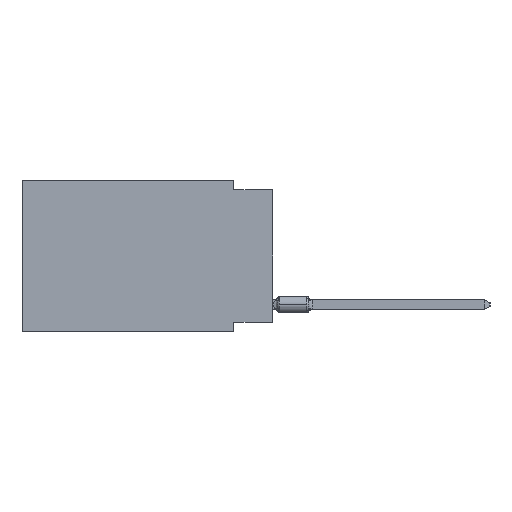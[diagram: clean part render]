
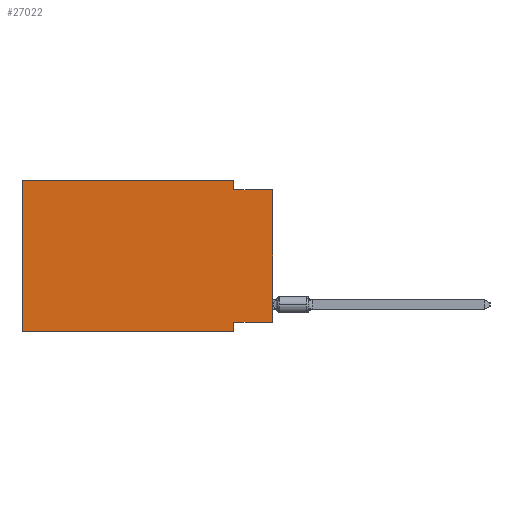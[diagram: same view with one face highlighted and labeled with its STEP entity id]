
A CAD part, left-side view. The second image highlights one B-rep face of the part: STEP entity #27022.
In plain terms, the highlighted planar face has unit normal (-1, 0, 0).
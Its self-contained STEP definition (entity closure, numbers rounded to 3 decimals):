
#645 = VERTEX_POINT ( 'NONE', #24655 ) ;
#1365 = CARTESIAN_POINT ( 'NONE',  ( 0., 0., -0.635 ) ) ;
#2185 = CARTESIAN_POINT ( 'NONE',  ( 0., 0., -0.635 ) ) ;
#3046 = LINE ( 'NONE', #20510, #38829 ) ;
#3589 = VERTEX_POINT ( 'NONE', #34357 ) ;
#4240 = DIRECTION ( 'NONE',  ( 0., 0., -1. ) ) ;
#5057 = DIRECTION ( 'NONE',  ( 0., -1., 0. ) ) ;
#5814 = LINE ( 'NONE', #32016, #23942 ) ;
#8572 = ORIENTED_EDGE ( 'NONE', *, *, #29410, .T. ) ;
#9543 = DIRECTION ( 'NONE',  ( 0., -1., 0. ) ) ;
#11314 = AXIS2_PLACEMENT_3D ( 'NONE', #19378, #15353, #42887 ) ;
#13610 = EDGE_LOOP ( 'NONE', ( #36660, #39043, #28194, #36894, #21786, #8572, #41357, #17095 ) ) ;
#13840 = CARTESIAN_POINT ( 'NONE',  ( 0., 16.383, 0. ) ) ;
#14112 = EDGE_CURVE ( 'NONE', #32189, #32602, #24391, .T. ) ;
#14381 = VECTOR ( 'NONE', #4240, 1000. ) ;
#15007 = DIRECTION ( 'NONE',  ( 0., 0., -1. ) ) ;
#15353 = DIRECTION ( 'NONE',  ( 1., 0., 0. ) ) ;
#16515 = CARTESIAN_POINT ( 'NONE',  ( 0., 2.54, -0.635 ) ) ;
#17095 = ORIENTED_EDGE ( 'NONE', *, *, #36737, .F. ) ;
#18501 = PLANE ( 'NONE',  #11314 ) ;
#18714 = DIRECTION ( 'NONE',  ( 0., 0., 1. ) ) ;
#19378 = CARTESIAN_POINT ( 'NONE',  ( 0., 16.383, 0. ) ) ;
#19677 = VECTOR ( 'NONE', #18714, 1000. ) ;
#20310 = VECTOR ( 'NONE', #5057, 1000. ) ;
#20337 = VECTOR ( 'NONE', #9543, 1000. ) ;
#20466 = VERTEX_POINT ( 'NONE', #32041 ) ;
#20510 = CARTESIAN_POINT ( 'NONE',  ( 0., 0., -9.271 ) ) ;
#21786 = ORIENTED_EDGE ( 'NONE', *, *, #35522, .F. ) ;
#22004 = DIRECTION ( 'NONE',  ( 0., -1., 0. ) ) ;
#22085 = LINE ( 'NONE', #35718, #20310 ) ;
#22220 = CARTESIAN_POINT ( 'NONE',  ( 0., 16.383, -9.906 ) ) ;
#23589 = VERTEX_POINT ( 'NONE', #1365 ) ;
#23942 = VECTOR ( 'NONE', #15007, 1000. ) ;
#24366 = VERTEX_POINT ( 'NONE', #29396 ) ;
#24391 = LINE ( 'NONE', #41410, #14381 ) ;
#24655 = CARTESIAN_POINT ( 'NONE',  ( 0., 16.383, -9.906 ) ) ;
#25864 = FACE_OUTER_BOUND ( 'NONE', #13610, .T. ) ;
#27022 = ADVANCED_FACE ( 'NONE', ( #25864 ), #18501, .F. ) ;
#27263 = LINE ( 'NONE', #13840, #30903 ) ;
#28077 = CARTESIAN_POINT ( 'NONE',  ( 0., 2.54, -9.271 ) ) ;
#28194 = ORIENTED_EDGE ( 'NONE', *, *, #14112, .F. ) ;
#28823 = EDGE_CURVE ( 'NONE', #38078, #20466, #5814, .T. ) ;
#29396 = CARTESIAN_POINT ( 'NONE',  ( 0., 16.383, 0. ) ) ;
#29410 = EDGE_CURVE ( 'NONE', #645, #20466, #42821, .T. ) ;
#30429 = EDGE_CURVE ( 'NONE', #32602, #23589, #36419, .T. ) ;
#30600 = EDGE_CURVE ( 'NONE', #3589, #23589, #42438, .T. ) ;
#30903 = VECTOR ( 'NONE', #37995, 1000. ) ;
#32016 = CARTESIAN_POINT ( 'NONE',  ( 0., 2.54, -9.906 ) ) ;
#32041 = CARTESIAN_POINT ( 'NONE',  ( 0., 2.54, -9.906 ) ) ;
#32189 = VERTEX_POINT ( 'NONE', #36528 ) ;
#32602 = VERTEX_POINT ( 'NONE', #16515 ) ;
#34357 = CARTESIAN_POINT ( 'NONE',  ( 0., 0., -9.271 ) ) ;
#35253 = CARTESIAN_POINT ( 'NONE',  ( 0., 0., 0. ) ) ;
#35522 = EDGE_CURVE ( 'NONE', #645, #24366, #27263, .T. ) ;
#35718 = CARTESIAN_POINT ( 'NONE',  ( 0., 16.383, 0. ) ) ;
#36419 = LINE ( 'NONE', #2185, #20337 ) ;
#36528 = CARTESIAN_POINT ( 'NONE',  ( 0., 2.54, 0. ) ) ;
#36660 = ORIENTED_EDGE ( 'NONE', *, *, #30600, .T. ) ;
#36737 = EDGE_CURVE ( 'NONE', #3589, #38078, #3046, .T. ) ;
#36854 = VECTOR ( 'NONE', #22004, 1000. ) ;
#36894 = ORIENTED_EDGE ( 'NONE', *, *, #38758, .F. ) ;
#37995 = DIRECTION ( 'NONE',  ( 0., 0., 1. ) ) ;
#38078 = VERTEX_POINT ( 'NONE', #28077 ) ;
#38758 = EDGE_CURVE ( 'NONE', #24366, #32189, #22085, .T. ) ;
#38829 = VECTOR ( 'NONE', #41094, 1000. ) ;
#39043 = ORIENTED_EDGE ( 'NONE', *, *, #30429, .F. ) ;
#41094 = DIRECTION ( 'NONE',  ( 0., 1., 0. ) ) ;
#41357 = ORIENTED_EDGE ( 'NONE', *, *, #28823, .F. ) ;
#41410 = CARTESIAN_POINT ( 'NONE',  ( 0., 2.54, 0. ) ) ;
#42438 = LINE ( 'NONE', #35253, #19677 ) ;
#42821 = LINE ( 'NONE', #22220, #36854 ) ;
#42887 = DIRECTION ( 'NONE',  ( 0., 0., -1. ) ) ;
